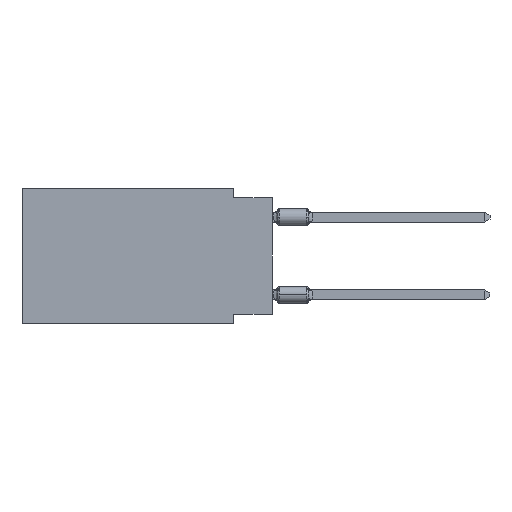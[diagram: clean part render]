
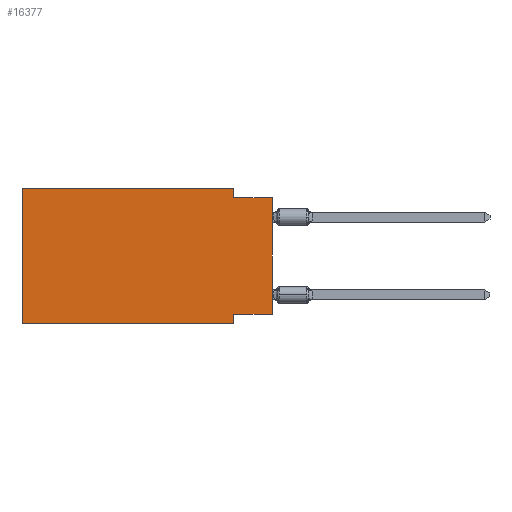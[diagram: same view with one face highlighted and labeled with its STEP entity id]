
A CAD part, left-side view. The second image highlights one B-rep face of the part: STEP entity #16377.
In plain terms, the highlighted planar face has unit normal (-1, 0, 0).
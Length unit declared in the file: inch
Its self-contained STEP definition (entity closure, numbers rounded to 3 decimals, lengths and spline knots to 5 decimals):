
#211 = ORIENTED_EDGE ( 'NONE', *, *, #20307, .T. ) ;
#231 = CARTESIAN_POINT ( 'NONE',  ( 0., 0.645, 0. ) ) ;
#412 = DIRECTION ( 'NONE',  ( 0., 0., -1. ) ) ;
#500 = DIRECTION ( 'NONE',  ( 0., 0., -1. ) ) ;
#597 = CARTESIAN_POINT ( 'NONE',  ( 0., 0., -0.325 ) ) ;
#1177 = VECTOR ( 'NONE', #19450, 39.37008 ) ;
#1326 = LINE ( 'NONE', #5079, #1177 ) ;
#1711 = VERTEX_POINT ( 'NONE', #2605 ) ;
#2177 = DIRECTION ( 'NONE',  ( 0., -1., 0. ) ) ;
#2441 = VERTEX_POINT ( 'NONE', #20084 ) ;
#2605 = CARTESIAN_POINT ( 'NONE',  ( 0., 0.645, -0.35 ) ) ;
#2663 = CARTESIAN_POINT ( 'NONE',  ( 0., 0.1, -0.35 ) ) ;
#2805 = CARTESIAN_POINT ( 'NONE',  ( 0., 0., -0.025 ) ) ;
#3248 = VERTEX_POINT ( 'NONE', #22727 ) ;
#3572 = DIRECTION ( 'NONE',  ( 0., -1., 0. ) ) ;
#3668 = VERTEX_POINT ( 'NONE', #231 ) ;
#3931 = LINE ( 'NONE', #16454, #23102 ) ;
#5071 = EDGE_CURVE ( 'NONE', #20950, #10666, #3931, .T. ) ;
#5079 = CARTESIAN_POINT ( 'NONE',  ( 0., 0.645, 0. ) ) ;
#5251 = ORIENTED_EDGE ( 'NONE', *, *, #8359, .F. ) ;
#5279 = VECTOR ( 'NONE', #2177, 39.37008 ) ;
#5514 = ORIENTED_EDGE ( 'NONE', *, *, #9231, .F. ) ;
#5550 = PLANE ( 'NONE',  #9411 ) ;
#6697 = DIRECTION ( 'NONE',  ( 0., 0., 1. ) ) ;
#7210 = CARTESIAN_POINT ( 'NONE',  ( 0., 0.645, -0.35 ) ) ;
#7465 = ORIENTED_EDGE ( 'NONE', *, *, #7751, .F. ) ;
#7751 = EDGE_CURVE ( 'NONE', #15542, #13611, #9238, .T. ) ;
#8238 = VECTOR ( 'NONE', #12415, 39.37008 ) ;
#8359 = EDGE_CURVE ( 'NONE', #3668, #3248, #16592, .T. ) ;
#9231 = EDGE_CURVE ( 'NONE', #1711, #3668, #1326, .T. ) ;
#9238 = LINE ( 'NONE', #18022, #8238 ) ;
#9411 = AXIS2_PLACEMENT_3D ( 'NONE', #11483, #9603, #17832 ) ;
#9586 = EDGE_CURVE ( 'NONE', #3248, #15542, #18266, .T. ) ;
#9603 = DIRECTION ( 'NONE',  ( 1., 0., 0. ) ) ;
#10011 = CARTESIAN_POINT ( 'NONE',  ( 0., 0.1, -0.325 ) ) ;
#10666 = VERTEX_POINT ( 'NONE', #2663 ) ;
#11133 = DIRECTION ( 'NONE',  ( 0., 1., 0. ) ) ;
#11375 = FACE_OUTER_BOUND ( 'NONE', #12552, .T. ) ;
#11483 = CARTESIAN_POINT ( 'NONE',  ( 0., 0.645, 0. ) ) ;
#12093 = LINE ( 'NONE', #15586, #18924 ) ;
#12415 = DIRECTION ( 'NONE',  ( 0., -1., 0. ) ) ;
#12552 = EDGE_LOOP ( 'NONE', ( #18611, #7465, #21704, #5251, #5514, #211, #14954, #22798 ) ) ;
#12662 = LINE ( 'NONE', #597, #20197 ) ;
#13217 = EDGE_CURVE ( 'NONE', #2441, #13611, #12093, .T. ) ;
#13611 = VERTEX_POINT ( 'NONE', #2805 ) ;
#14954 = ORIENTED_EDGE ( 'NONE', *, *, #5071, .F. ) ;
#15094 = EDGE_CURVE ( 'NONE', #2441, #20950, #12662, .T. ) ;
#15542 = VERTEX_POINT ( 'NONE', #16274 ) ;
#15586 = CARTESIAN_POINT ( 'NONE',  ( 0., 0., 0. ) ) ;
#15786 = VECTOR ( 'NONE', #500, 39.37008 ) ;
#16274 = CARTESIAN_POINT ( 'NONE',  ( 0., 0.1, -0.025 ) ) ;
#16377 = ADVANCED_FACE ( 'NONE', ( #11375 ), #5550, .F. ) ;
#16454 = CARTESIAN_POINT ( 'NONE',  ( 0., 0.1, -0.35 ) ) ;
#16471 = CARTESIAN_POINT ( 'NONE',  ( 0., 0.645, 0. ) ) ;
#16538 = CARTESIAN_POINT ( 'NONE',  ( 0., 0.1, 0. ) ) ;
#16592 = LINE ( 'NONE', #16471, #5279 ) ;
#17832 = DIRECTION ( 'NONE',  ( 0., 0., -1. ) ) ;
#17912 = VECTOR ( 'NONE', #3572, 39.37008 ) ;
#18022 = CARTESIAN_POINT ( 'NONE',  ( 0., 0., -0.025 ) ) ;
#18266 = LINE ( 'NONE', #16538, #15786 ) ;
#18611 = ORIENTED_EDGE ( 'NONE', *, *, #13217, .T. ) ;
#18924 = VECTOR ( 'NONE', #6697, 39.37008 ) ;
#19450 = DIRECTION ( 'NONE',  ( 0., 0., 1. ) ) ;
#19937 = LINE ( 'NONE', #7210, #17912 ) ;
#20084 = CARTESIAN_POINT ( 'NONE',  ( 0., 0., -0.325 ) ) ;
#20197 = VECTOR ( 'NONE', #11133, 39.37008 ) ;
#20307 = EDGE_CURVE ( 'NONE', #1711, #10666, #19937, .T. ) ;
#20950 = VERTEX_POINT ( 'NONE', #10011 ) ;
#21704 = ORIENTED_EDGE ( 'NONE', *, *, #9586, .F. ) ;
#22727 = CARTESIAN_POINT ( 'NONE',  ( 0., 0.1, 0. ) ) ;
#22798 = ORIENTED_EDGE ( 'NONE', *, *, #15094, .F. ) ;
#23102 = VECTOR ( 'NONE', #412, 39.37008 ) ;
